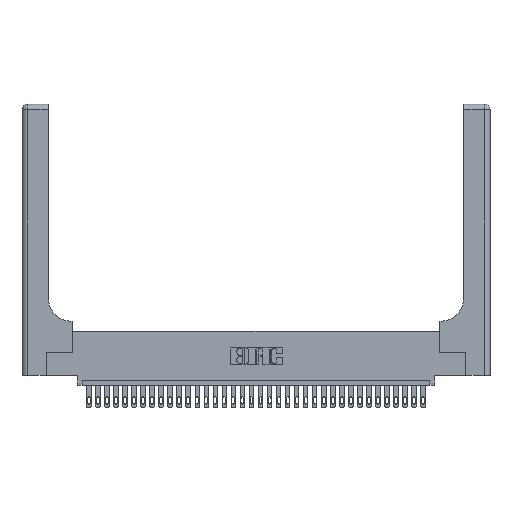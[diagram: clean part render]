
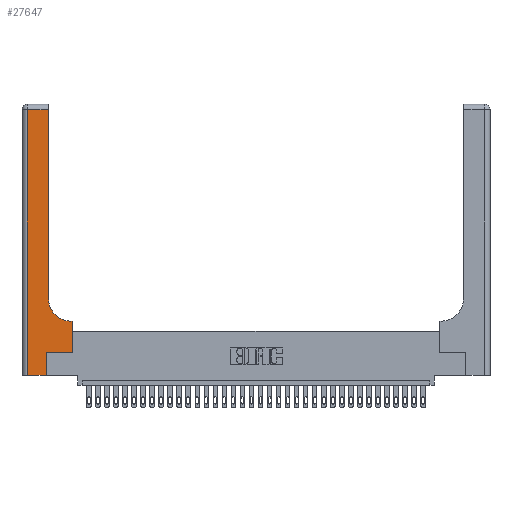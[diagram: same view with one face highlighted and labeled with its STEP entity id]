
A CAD part, top view. The second image highlights one B-rep face of the part: STEP entity #27647.
In plain terms, the highlighted planar face has unit normal (0, 0, 1).
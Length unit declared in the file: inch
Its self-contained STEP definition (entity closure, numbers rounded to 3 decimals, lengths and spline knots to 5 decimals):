
#255 = ORIENTED_EDGE ( 'NONE', *, *, #17162, .T. ) ;
#1843 = CARTESIAN_POINT ( 'NONE',  ( 0.2915, 3., 0.37 ) ) ;
#1882 = DIRECTION ( 'NONE',  ( 0., 0., -1. ) ) ;
#2137 = ORIENTED_EDGE ( 'NONE', *, *, #22394, .T. ) ;
#2294 = DIRECTION ( 'NONE',  ( -1., 0., 0. ) ) ;
#2543 = LINE ( 'NONE', #24957, #4557 ) ;
#2698 = LINE ( 'NONE', #29713, #10131 ) ;
#2932 = DIRECTION ( 'NONE',  ( -1., 0., 0. ) ) ;
#3189 = VERTEX_POINT ( 'NONE', #19536 ) ;
#3264 = CARTESIAN_POINT ( 'NONE',  ( 0.5415, 0.6, 0.37 ) ) ;
#3431 = DIRECTION ( 'NONE',  ( 0., 0., -1. ) ) ;
#3757 = AXIS2_PLACEMENT_3D ( 'NONE', #28569, #1882, #15306 ) ;
#3866 = VERTEX_POINT ( 'NONE', #8373 ) ;
#4008 = EDGE_LOOP ( 'NONE', ( #29630, #26407, #2137, #19174, #33062, #12054, #255, #29661, #5590 ) ) ;
#4182 = AXIS2_PLACEMENT_3D ( 'NONE', #14101, #3431, #27236 ) ;
#4367 = EDGE_CURVE ( 'NONE', #20645, #17310, #17795, .T. ) ;
#4557 = VECTOR ( 'NONE', #19936, 39.37008 ) ;
#4919 = CARTESIAN_POINT ( 'NONE',  ( 0.269, 0.25, 0.37 ) ) ;
#5257 = VERTEX_POINT ( 'NONE', #17872 ) ;
#5590 = ORIENTED_EDGE ( 'NONE', *, *, #11337, .T. ) ;
#5966 = LINE ( 'NONE', #4919, #33396 ) ;
#6871 = FACE_OUTER_BOUND ( 'NONE', #4008, .T. ) ;
#7059 = VECTOR ( 'NONE', #25017, 39.37008 ) ;
#7112 = CIRCLE ( 'NONE', #4182, 0.25 ) ;
#7410 = VECTOR ( 'NONE', #34113, 39.37008 ) ;
#8373 = CARTESIAN_POINT ( 'NONE',  ( 0.2915, 0.85, 0.37 ) ) ;
#9025 = DIRECTION ( 'NONE',  ( 0., -1., 0. ) ) ;
#9125 = LINE ( 'NONE', #28744, #14541 ) ;
#10131 = VECTOR ( 'NONE', #9025, 39.37008 ) ;
#10437 = VERTEX_POINT ( 'NONE', #3264 ) ;
#11337 = EDGE_CURVE ( 'NONE', #10437, #3866, #7112, .T. ) ;
#12054 = ORIENTED_EDGE ( 'NONE', *, *, #28989, .T. ) ;
#13780 = VERTEX_POINT ( 'NONE', #31546 ) ;
#14101 = CARTESIAN_POINT ( 'NONE',  ( 0.5415, 0.85, 0.37 ) ) ;
#14224 = VECTOR ( 'NONE', #2932, 39.37008 ) ;
#14541 = VECTOR ( 'NONE', #2294, 39.37008 ) ;
#14911 = VERTEX_POINT ( 'NONE', #24202 ) ;
#15306 = DIRECTION ( 'NONE',  ( -1., 0., 0. ) ) ;
#15690 = EDGE_CURVE ( 'NONE', #5257, #13780, #31294, .T. ) ;
#15866 = CARTESIAN_POINT ( 'NONE',  ( 0.269, 0., 0.37 ) ) ;
#16339 = EDGE_CURVE ( 'NONE', #3866, #5257, #30815, .T. ) ;
#16772 = DIRECTION ( 'NONE',  ( 1., 0., 0. ) ) ;
#17162 = EDGE_CURVE ( 'NONE', #14911, #25232, #2543, .T. ) ;
#17290 = CARTESIAN_POINT ( 'NONE',  ( 0.5585, 0.6, 0.37 ) ) ;
#17310 = VERTEX_POINT ( 'NONE', #31798 ) ;
#17757 = CARTESIAN_POINT ( 'NONE',  ( 0.269, 0., 0.37 ) ) ;
#17795 = LINE ( 'NONE', #15866, #7410 ) ;
#17872 = CARTESIAN_POINT ( 'NONE',  ( 0.2915, 2.94, 0.37 ) ) ;
#19174 = ORIENTED_EDGE ( 'NONE', *, *, #34380, .T. ) ;
#19536 = CARTESIAN_POINT ( 'NONE',  ( 0.06, 0., 0.37 ) ) ;
#19936 = DIRECTION ( 'NONE',  ( 0., 1., 0. ) ) ;
#20645 = VERTEX_POINT ( 'NONE', #17757 ) ;
#22394 = EDGE_CURVE ( 'NONE', #13780, #3189, #2698, .T. ) ;
#24202 = CARTESIAN_POINT ( 'NONE',  ( 0.5585, 0.25, 0.37 ) ) ;
#24520 = CARTESIAN_POINT ( 'NONE',  ( 0., 2.94, 0.37 ) ) ;
#24957 = CARTESIAN_POINT ( 'NONE',  ( 0.5585, 0.25, 0.37 ) ) ;
#25017 = DIRECTION ( 'NONE',  ( 0., 1., 0. ) ) ;
#25232 = VERTEX_POINT ( 'NONE', #17290 ) ;
#25905 = PLANE ( 'NONE',  #3757 ) ;
#26407 = ORIENTED_EDGE ( 'NONE', *, *, #15690, .T. ) ;
#26933 = VECTOR ( 'NONE', #16772, 39.37008 ) ;
#27236 = DIRECTION ( 'NONE',  ( 1., 0., 0. ) ) ;
#27647 = ADVANCED_FACE ( 'NONE', ( #6871 ), #25905, .F. ) ;
#27785 = LINE ( 'NONE', #32519, #26933 ) ;
#28569 = CARTESIAN_POINT ( 'NONE',  ( 0., 3., 0.37 ) ) ;
#28744 = CARTESIAN_POINT ( 'NONE',  ( 0.2915, 0.6, 0.37 ) ) ;
#28989 = EDGE_CURVE ( 'NONE', #17310, #14911, #5966, .T. ) ;
#29630 = ORIENTED_EDGE ( 'NONE', *, *, #16339, .T. ) ;
#29661 = ORIENTED_EDGE ( 'NONE', *, *, #33411, .T. ) ;
#29713 = CARTESIAN_POINT ( 'NONE',  ( 0.06, 3., 0.37 ) ) ;
#30815 = LINE ( 'NONE', #1843, #7059 ) ;
#31294 = LINE ( 'NONE', #24520, #14224 ) ;
#31546 = CARTESIAN_POINT ( 'NONE',  ( 0.06, 2.94, 0.37 ) ) ;
#31798 = CARTESIAN_POINT ( 'NONE',  ( 0.269, 0.25, 0.37 ) ) ;
#32519 = CARTESIAN_POINT ( 'NONE',  ( 0., 0., 0.37 ) ) ;
#33062 = ORIENTED_EDGE ( 'NONE', *, *, #4367, .T. ) ;
#33396 = VECTOR ( 'NONE', #34063, 39.37008 ) ;
#33411 = EDGE_CURVE ( 'NONE', #25232, #10437, #9125, .T. ) ;
#34063 = DIRECTION ( 'NONE',  ( 1., 0., 0. ) ) ;
#34113 = DIRECTION ( 'NONE',  ( 0., 1., 0. ) ) ;
#34380 = EDGE_CURVE ( 'NONE', #3189, #20645, #27785, .T. ) ;
